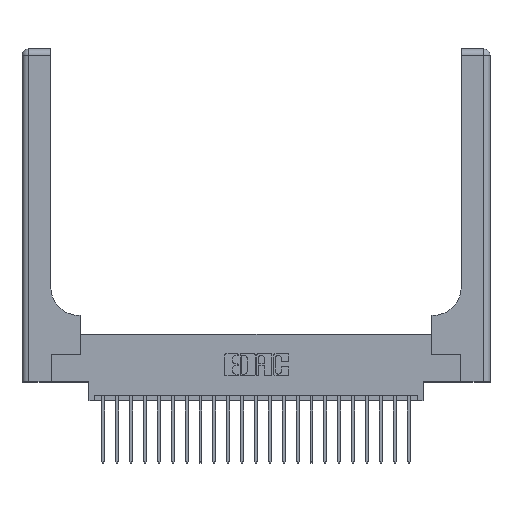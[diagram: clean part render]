
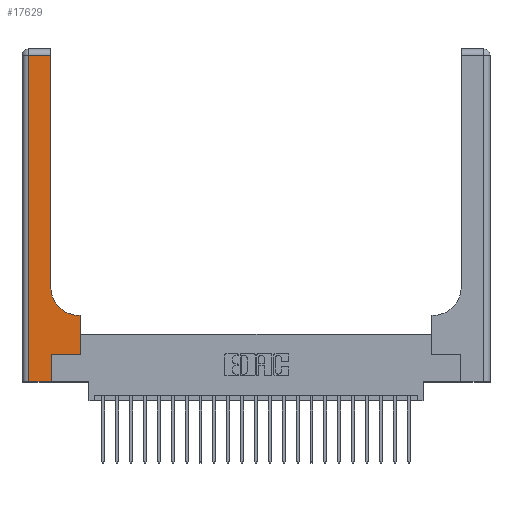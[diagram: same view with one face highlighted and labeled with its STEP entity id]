
A CAD part, top view. The second image highlights one B-rep face of the part: STEP entity #17629.
In plain terms, the highlighted planar face has unit normal (0, 0, 1).
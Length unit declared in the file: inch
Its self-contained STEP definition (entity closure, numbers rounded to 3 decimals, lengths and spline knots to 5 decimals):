
#355 = VERTEX_POINT ( 'NONE', #11896 ) ;
#1262 = DIRECTION ( 'NONE',  ( -1., 0., 0. ) ) ;
#1359 = LINE ( 'NONE', #4913, #7519 ) ;
#1425 = DIRECTION ( 'NONE',  ( 0., 1., 0. ) ) ;
#1487 = CARTESIAN_POINT ( 'NONE',  ( 0., 0., 0.37 ) ) ;
#1699 = LINE ( 'NONE', #17766, #11632 ) ;
#2119 = CARTESIAN_POINT ( 'NONE',  ( 0.26, 0.85, 0.37 ) ) ;
#2136 = AXIS2_PLACEMENT_3D ( 'NONE', #9365, #14810, #16692 ) ;
#2316 = EDGE_CURVE ( 'NONE', #13123, #355, #1699, .T. ) ;
#2465 = DIRECTION ( 'NONE',  ( -1., 0., 0. ) ) ;
#3254 = VERTEX_POINT ( 'NONE', #7197 ) ;
#3385 = ORIENTED_EDGE ( 'NONE', *, *, #2316, .T. ) ;
#3397 = DIRECTION ( 'NONE',  ( 1., 0., 0. ) ) ;
#3898 = VERTEX_POINT ( 'NONE', #8105 ) ;
#4028 = EDGE_CURVE ( 'NONE', #9293, #4201, #1359, .T. ) ;
#4201 = VERTEX_POINT ( 'NONE', #11593 ) ;
#4243 = CARTESIAN_POINT ( 'NONE',  ( 0., 2.94, 0.37 ) ) ;
#4913 = CARTESIAN_POINT ( 'NONE',  ( 0.06, 3., 0.37 ) ) ;
#5218 = EDGE_CURVE ( 'NONE', #8055, #3898, #23171, .T. ) ;
#5327 = CARTESIAN_POINT ( 'NONE',  ( 0.528, 0.25, 0.37 ) ) ;
#5967 = VERTEX_POINT ( 'NONE', #9971 ) ;
#6055 = CARTESIAN_POINT ( 'NONE',  ( 0.528, 0.25, 0.37 ) ) ;
#6291 = CIRCLE ( 'NONE', #2136, 0.25 ) ;
#6642 = CARTESIAN_POINT ( 'NONE',  ( 0.06, 2.94, 0.37 ) ) ;
#6917 = LINE ( 'NONE', #1487, #18660 ) ;
#7111 = VECTOR ( 'NONE', #2465, 39.37008 ) ;
#7137 = ORIENTED_EDGE ( 'NONE', *, *, #20375, .T. ) ;
#7197 = CARTESIAN_POINT ( 'NONE',  ( 0.265, 0.25, 0.37 ) ) ;
#7427 = EDGE_CURVE ( 'NONE', #4201, #5967, #6917, .T. ) ;
#7466 = VECTOR ( 'NONE', #3397, 39.37008 ) ;
#7519 = VECTOR ( 'NONE', #19545, 39.37008 ) ;
#7878 = ORIENTED_EDGE ( 'NONE', *, *, #7427, .T. ) ;
#8033 = LINE ( 'NONE', #11941, #12813 ) ;
#8055 = VERTEX_POINT ( 'NONE', #2119 ) ;
#8105 = CARTESIAN_POINT ( 'NONE',  ( 0.26, 2.94, 0.37 ) ) ;
#8186 = LINE ( 'NONE', #6055, #13423 ) ;
#8347 = ORIENTED_EDGE ( 'NONE', *, *, #14897, .T. ) ;
#9265 = EDGE_CURVE ( 'NONE', #20060, #13123, #8186, .T. ) ;
#9293 = VERTEX_POINT ( 'NONE', #6642 ) ;
#9365 = CARTESIAN_POINT ( 'NONE',  ( 0.51, 0.85, 0.37 ) ) ;
#9971 = CARTESIAN_POINT ( 'NONE',  ( 0.265, 0., 0.37 ) ) ;
#10110 = DIRECTION ( 'NONE',  ( 0., 0., -1. ) ) ;
#10399 = CARTESIAN_POINT ( 'NONE',  ( 0.26, 3., 0.37 ) ) ;
#10484 = VECTOR ( 'NONE', #1425, 39.37008 ) ;
#11577 = DIRECTION ( 'NONE',  ( 0., 1., 0. ) ) ;
#11593 = CARTESIAN_POINT ( 'NONE',  ( 0.06, 0., 0.37 ) ) ;
#11632 = VECTOR ( 'NONE', #14346, 39.37008 ) ;
#11896 = CARTESIAN_POINT ( 'NONE',  ( 0.51, 0.6, 0.37 ) ) ;
#11938 = LINE ( 'NONE', #4243, #7111 ) ;
#11941 = CARTESIAN_POINT ( 'NONE',  ( 0.265, 0., 0.37 ) ) ;
#12153 = EDGE_LOOP ( 'NONE', ( #12482, #20398, #16944, #7878, #7137, #15051, #13095, #3385, #8347 ) ) ;
#12482 = ORIENTED_EDGE ( 'NONE', *, *, #5218, .T. ) ;
#12499 = LINE ( 'NONE', #12610, #7466 ) ;
#12592 = DIRECTION ( 'NONE',  ( 1., 0., 0. ) ) ;
#12610 = CARTESIAN_POINT ( 'NONE',  ( 0.265, 0.25, 0.37 ) ) ;
#12813 = VECTOR ( 'NONE', #11577, 39.37008 ) ;
#13095 = ORIENTED_EDGE ( 'NONE', *, *, #9265, .T. ) ;
#13123 = VERTEX_POINT ( 'NONE', #22428 ) ;
#13151 = DIRECTION ( 'NONE',  ( 0., 1., 0. ) ) ;
#13423 = VECTOR ( 'NONE', #13151, 39.37008 ) ;
#14346 = DIRECTION ( 'NONE',  ( -1., 0., 0. ) ) ;
#14810 = DIRECTION ( 'NONE',  ( 0., 0., -1. ) ) ;
#14897 = EDGE_CURVE ( 'NONE', #355, #8055, #6291, .T. ) ;
#15051 = ORIENTED_EDGE ( 'NONE', *, *, #16261, .T. ) ;
#15551 = FACE_OUTER_BOUND ( 'NONE', #12153, .T. ) ;
#16261 = EDGE_CURVE ( 'NONE', #3254, #20060, #12499, .T. ) ;
#16692 = DIRECTION ( 'NONE',  ( 1., 0., 0. ) ) ;
#16944 = ORIENTED_EDGE ( 'NONE', *, *, #4028, .T. ) ;
#17629 = ADVANCED_FACE ( 'NONE', ( #15551 ), #22531, .F. ) ;
#17766 = CARTESIAN_POINT ( 'NONE',  ( 0.26, 0.6, 0.37 ) ) ;
#18660 = VECTOR ( 'NONE', #12592, 39.37008 ) ;
#19103 = EDGE_CURVE ( 'NONE', #3898, #9293, #11938, .T. ) ;
#19545 = DIRECTION ( 'NONE',  ( 0., -1., 0. ) ) ;
#20060 = VERTEX_POINT ( 'NONE', #5327 ) ;
#20344 = AXIS2_PLACEMENT_3D ( 'NONE', #20880, #10110, #1262 ) ;
#20375 = EDGE_CURVE ( 'NONE', #5967, #3254, #8033, .T. ) ;
#20398 = ORIENTED_EDGE ( 'NONE', *, *, #19103, .T. ) ;
#20880 = CARTESIAN_POINT ( 'NONE',  ( 0., 3., 0.37 ) ) ;
#22428 = CARTESIAN_POINT ( 'NONE',  ( 0.528, 0.6, 0.37 ) ) ;
#22531 = PLANE ( 'NONE',  #20344 ) ;
#23171 = LINE ( 'NONE', #10399, #10484 ) ;
